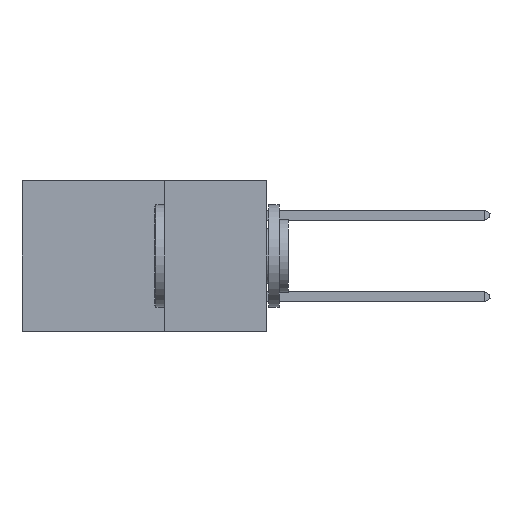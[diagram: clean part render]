
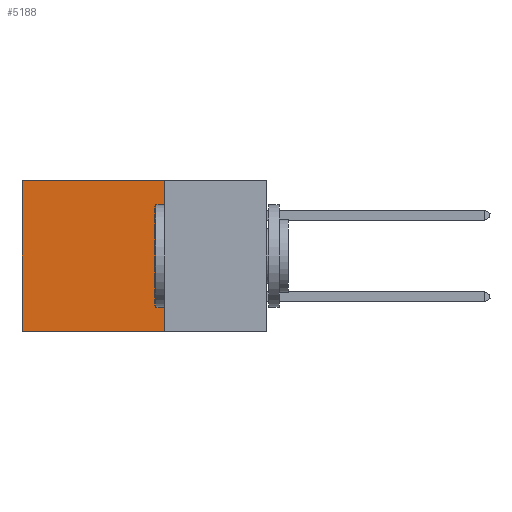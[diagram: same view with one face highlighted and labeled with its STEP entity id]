
A CAD part, left-side view. The second image highlights one B-rep face of the part: STEP entity #5188.
In plain terms, the highlighted planar face has unit normal (-1, 0, 0).
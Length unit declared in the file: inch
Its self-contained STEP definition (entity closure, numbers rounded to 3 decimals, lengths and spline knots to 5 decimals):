
#570 = ORIENTED_EDGE ( 'NONE', *, *, #5544, .F. ) ;
#825 = CARTESIAN_POINT ( 'NONE',  ( 0.2875, 0.25, 0. ) ) ;
#866 = DIRECTION ( 'NONE',  ( 0., 0., -1. ) ) ;
#1003 = DIRECTION ( 'NONE',  ( 0., 0., -1. ) ) ;
#1681 = VERTEX_POINT ( 'NONE', #13196 ) ;
#1885 = EDGE_CURVE ( 'NONE', #1681, #9804, #6402, .T. ) ;
#2148 = CARTESIAN_POINT ( 'NONE',  ( 0.2875, 0.6, 0. ) ) ;
#2613 = CARTESIAN_POINT ( 'NONE',  ( 0.2875, 0.25, -0.37 ) ) ;
#2620 = DIRECTION ( 'NONE',  ( 0., 1., 0. ) ) ;
#2878 = VECTOR ( 'NONE', #1003, 39.37008 ) ;
#3194 = CARTESIAN_POINT ( 'NONE',  ( 0.2875, 0.6, -0.37 ) ) ;
#3338 = AXIS2_PLACEMENT_3D ( 'NONE', #7480, #7446, #7426 ) ;
#3658 = VECTOR ( 'NONE', #13436, 39.37008 ) ;
#3687 = VECTOR ( 'NONE', #866, 39.37008 ) ;
#4099 = EDGE_CURVE ( 'NONE', #4995, #12095, #13291, .T. ) ;
#4297 = ORIENTED_EDGE ( 'NONE', *, *, #4099, .F. ) ;
#4995 = VERTEX_POINT ( 'NONE', #11253 ) ;
#5188 = ADVANCED_FACE ( 'NONE', ( #8527 ), #7731, .F. ) ;
#5351 = ORIENTED_EDGE ( 'NONE', *, *, #1885, .T. ) ;
#5544 = EDGE_CURVE ( 'NONE', #1681, #4995, #6757, .T. ) ;
#5658 = ORIENTED_EDGE ( 'NONE', *, *, #12137, .T. ) ;
#6402 = LINE ( 'NONE', #13234, #3658 ) ;
#6757 = LINE ( 'NONE', #825, #3687 ) ;
#6964 = EDGE_LOOP ( 'NONE', ( #5658, #4297, #570, #5351 ) ) ;
#7426 = DIRECTION ( 'NONE',  ( 0., 0., -1. ) ) ;
#7446 = DIRECTION ( 'NONE',  ( 1., 0., 0. ) ) ;
#7480 = CARTESIAN_POINT ( 'NONE',  ( 0.2875, 0.25, 0. ) ) ;
#7731 = PLANE ( 'NONE',  #3338 ) ;
#8317 = LINE ( 'NONE', #2148, #2878 ) ;
#8527 = FACE_OUTER_BOUND ( 'NONE', #6964, .T. ) ;
#9804 = VERTEX_POINT ( 'NONE', #13482 ) ;
#10881 = VECTOR ( 'NONE', #2620, 39.37008 ) ;
#11253 = CARTESIAN_POINT ( 'NONE',  ( 0.2875, 0.25, -0.37 ) ) ;
#12095 = VERTEX_POINT ( 'NONE', #3194 ) ;
#12137 = EDGE_CURVE ( 'NONE', #9804, #12095, #8317, .T. ) ;
#13196 = CARTESIAN_POINT ( 'NONE',  ( 0.2875, 0.25, 0. ) ) ;
#13234 = CARTESIAN_POINT ( 'NONE',  ( 0.2875, 0.25, 0. ) ) ;
#13291 = LINE ( 'NONE', #2613, #10881 ) ;
#13436 = DIRECTION ( 'NONE',  ( 0., 1., 0. ) ) ;
#13482 = CARTESIAN_POINT ( 'NONE',  ( 0.2875, 0.6, 0. ) ) ;
